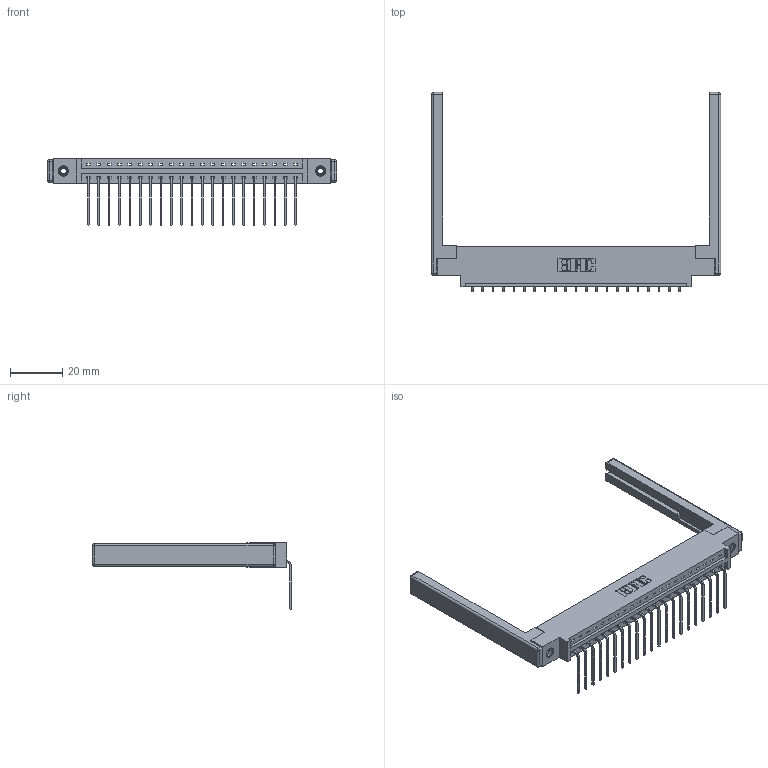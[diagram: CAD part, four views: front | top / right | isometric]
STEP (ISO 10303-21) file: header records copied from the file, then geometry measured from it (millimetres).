
FILE_DESCRIPTION (( 'STEP AP203' ), '1' );
FILE_NAME ('387-021-559-668.STEP', '2019-10-03T00:38:54', ( '' ), ( '' ), 'SwSTEP 2.0', 'SolidWorks 2016', '' );
FILE_SCHEMA (( 'CONFIG_CONTROL_DESIGN' ));
Length unit declared in the file: inch
Products named in the file (5): 345-250-001_345-250-001-102; 337 Part_0.170 Offset - 0.156 Dia-TI; 387-021-559-668; 345-292-001_558 559 Tail - 1; 307-220-068
Assembly tree (26 placements, depth 2):
  387-021-559-668
    337 Part_0.170 Offset - 0.156 Dia-TI
    345-292-001_558 559 Tail - 1  x21
    345-250-001_345-250-001-102  x2
    307-220-068  x2
Bounding box: 110.64 x 76.14 x 25.53 mm (x, y, z)
Volume: 15580.3 mm3; surface area: 16064.7 mm2
Topology: 26 solids, 26 shells, 1616 faces, 4787 edges, 3142 vertices
Faces by surface type: plane 1170, cylinder 422, cone 12, sphere 8, torus 4
Entity records: 21302 total; most frequent: CARTESIAN_POINT 3666, ORIENTED_EDGE 3612, DIRECTION 3202, EDGE_CURVE 1806, LINE 1628, VECTOR 1628, VERTEX_POINT 1194, AXIS2_PLACEMENT_3D 787
